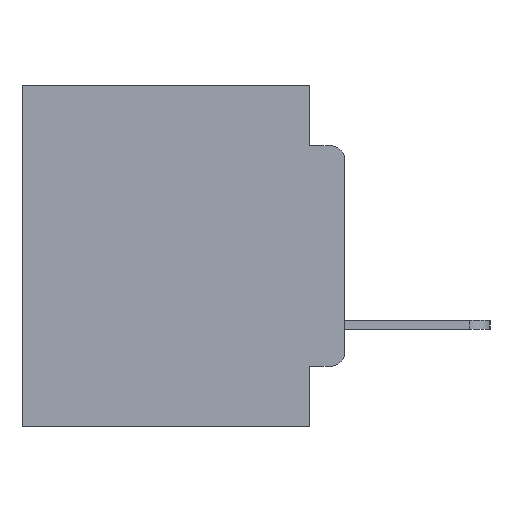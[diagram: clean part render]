
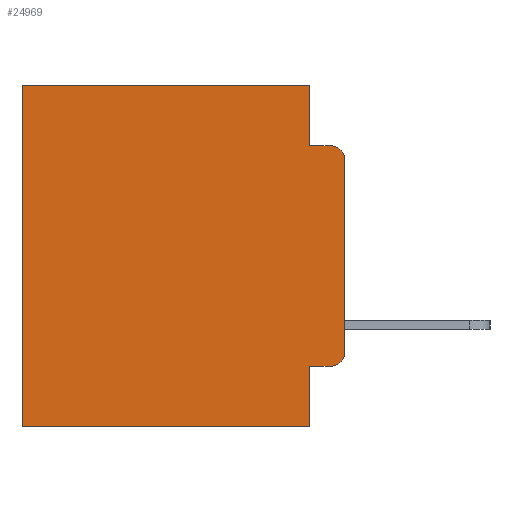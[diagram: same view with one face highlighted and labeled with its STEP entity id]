
A CAD part, left-side view. The second image highlights one B-rep face of the part: STEP entity #24969.
In plain terms, the highlighted planar face has unit normal (-1, 0, 0).
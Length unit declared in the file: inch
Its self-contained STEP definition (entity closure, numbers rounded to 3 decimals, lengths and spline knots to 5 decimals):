
#484 = CARTESIAN_POINT ( 'NONE',  ( 0.298, 0., -0.3915 ) ) ;
#609 = LINE ( 'NONE', #15113, #22962 ) ;
#954 = ORIENTED_EDGE ( 'NONE', *, *, #9728, .F. ) ;
#973 = CARTESIAN_POINT ( 'NONE',  ( 0.298, 0., 0. ) ) ;
#975 = EDGE_CURVE ( 'NONE', #1327, #17367, #3357, .T. ) ;
#1094 = LINE ( 'NONE', #25729, #12851 ) ;
#1327 = VERTEX_POINT ( 'NONE', #2108 ) ;
#1546 = CARTESIAN_POINT ( 'NONE',  ( 0.298, 0.051, -0.0885 ) ) ;
#2009 = EDGE_CURVE ( 'NONE', #8742, #11650, #5872, .T. ) ;
#2108 = CARTESIAN_POINT ( 'NONE',  ( 0.298, 0.473, 0. ) ) ;
#2180 = DIRECTION ( 'NONE',  ( -1., 0., 0. ) ) ;
#2583 = EDGE_CURVE ( 'NONE', #17834, #11650, #7219, .T. ) ;
#2671 = VECTOR ( 'NONE', #15167, 39.37008 ) ;
#2729 = VECTOR ( 'NONE', #8973, 39.37008 ) ;
#2906 = EDGE_CURVE ( 'NONE', #24728, #1327, #5493, .T. ) ;
#3357 = LINE ( 'NONE', #18942, #2729 ) ;
#3561 = ORIENTED_EDGE ( 'NONE', *, *, #2906, .T. ) ;
#4038 = CARTESIAN_POINT ( 'NONE',  ( 0.298, 0.051, -0.4115 ) ) ;
#5493 = LINE ( 'NONE', #973, #15902 ) ;
#5729 = DIRECTION ( 'NONE',  ( 0., 0., -1. ) ) ;
#5872 = LINE ( 'NONE', #25750, #15627 ) ;
#6986 = EDGE_LOOP ( 'NONE', ( #23642, #17729, #954, #14649, #3561, #11754, #18339, #25602, #8555, #21594 ) ) ;
#7070 = DIRECTION ( 'NONE',  ( 1., 0., 0. ) ) ;
#7219 = CIRCLE ( 'NONE', #7314, 0.02 ) ;
#7314 = AXIS2_PLACEMENT_3D ( 'NONE', #21985, #21525, #8734 ) ;
#8555 = ORIENTED_EDGE ( 'NONE', *, *, #23397, .T. ) ;
#8585 = DIRECTION ( 'NONE',  ( 0., -1., 0. ) ) ;
#8734 = DIRECTION ( 'NONE',  ( 0., 0., -1. ) ) ;
#8742 = VERTEX_POINT ( 'NONE', #20055 ) ;
#8872 = CARTESIAN_POINT ( 'NONE',  ( 0.298, 0.051, 0. ) ) ;
#8973 = DIRECTION ( 'NONE',  ( 0., 0., -1. ) ) ;
#9070 = EDGE_CURVE ( 'NONE', #24728, #11691, #13868, .T. ) ;
#9728 = EDGE_CURVE ( 'NONE', #11691, #14777, #12380, .T. ) ;
#11650 = VERTEX_POINT ( 'NONE', #484 ) ;
#11691 = VERTEX_POINT ( 'NONE', #25929 ) ;
#11754 = ORIENTED_EDGE ( 'NONE', *, *, #975, .T. ) ;
#12145 = DIRECTION ( 'NONE',  ( 0., 0., -1. ) ) ;
#12380 = LINE ( 'NONE', #1546, #22960 ) ;
#12495 = CARTESIAN_POINT ( 'NONE',  ( 0.298, 0.02, -0.0885 ) ) ;
#12851 = VECTOR ( 'NONE', #21689, 39.37008 ) ;
#13144 = CARTESIAN_POINT ( 'NONE',  ( 0.298, 0.051, -0.4115 ) ) ;
#13265 = VERTEX_POINT ( 'NONE', #4038 ) ;
#13487 = EDGE_CURVE ( 'NONE', #20129, #17367, #1094, .T. ) ;
#13746 = LINE ( 'NONE', #13144, #2671 ) ;
#13868 = LINE ( 'NONE', #8872, #19118 ) ;
#14029 = AXIS2_PLACEMENT_3D ( 'NONE', #19245, #7070, #21231 ) ;
#14601 = CARTESIAN_POINT ( 'NONE',  ( 0.298, 0.02, -0.1085 ) ) ;
#14649 = ORIENTED_EDGE ( 'NONE', *, *, #9070, .F. ) ;
#14777 = VERTEX_POINT ( 'NONE', #12495 ) ;
#15113 = CARTESIAN_POINT ( 'NONE',  ( 0.298, 0.051, 0. ) ) ;
#15167 = DIRECTION ( 'NONE',  ( 0., -1., 0. ) ) ;
#15296 = PLANE ( 'NONE',  #14029 ) ;
#15627 = VECTOR ( 'NONE', #12145, 39.37008 ) ;
#15902 = VECTOR ( 'NONE', #20746, 39.37008 ) ;
#16587 = DIRECTION ( 'NONE',  ( 0., 0., -1. ) ) ;
#16602 = CARTESIAN_POINT ( 'NONE',  ( 0.298, 0.051, 0. ) ) ;
#16802 = CARTESIAN_POINT ( 'NONE',  ( 0.298, 0.051, -0.5 ) ) ;
#16977 = EDGE_CURVE ( 'NONE', #13265, #20129, #609, .T. ) ;
#17367 = VERTEX_POINT ( 'NONE', #23023 ) ;
#17729 = ORIENTED_EDGE ( 'NONE', *, *, #21370, .T. ) ;
#17834 = VERTEX_POINT ( 'NONE', #20975 ) ;
#18201 = CIRCLE ( 'NONE', #18801, 0.02 ) ;
#18339 = ORIENTED_EDGE ( 'NONE', *, *, #13487, .F. ) ;
#18801 = AXIS2_PLACEMENT_3D ( 'NONE', #14601, #2180, #16587 ) ;
#18942 = CARTESIAN_POINT ( 'NONE',  ( 0.298, 0.473, 0. ) ) ;
#19118 = VECTOR ( 'NONE', #21144, 39.37008 ) ;
#19245 = CARTESIAN_POINT ( 'NONE',  ( 0.298, 0., 0. ) ) ;
#20055 = CARTESIAN_POINT ( 'NONE',  ( 0.298, 0., -0.1085 ) ) ;
#20129 = VERTEX_POINT ( 'NONE', #16802 ) ;
#20499 = FACE_OUTER_BOUND ( 'NONE', #6986, .T. ) ;
#20746 = DIRECTION ( 'NONE',  ( 0., 1., 0. ) ) ;
#20975 = CARTESIAN_POINT ( 'NONE',  ( 0.298, 0.02, -0.4115 ) ) ;
#21144 = DIRECTION ( 'NONE',  ( 0., 0., -1. ) ) ;
#21231 = DIRECTION ( 'NONE',  ( 0., 0., -1. ) ) ;
#21370 = EDGE_CURVE ( 'NONE', #8742, #14777, #18201, .T. ) ;
#21525 = DIRECTION ( 'NONE',  ( -1., 0., 0. ) ) ;
#21594 = ORIENTED_EDGE ( 'NONE', *, *, #2583, .T. ) ;
#21689 = DIRECTION ( 'NONE',  ( 0., 1., 0. ) ) ;
#21985 = CARTESIAN_POINT ( 'NONE',  ( 0.298, 0.02, -0.3915 ) ) ;
#22960 = VECTOR ( 'NONE', #8585, 39.37008 ) ;
#22962 = VECTOR ( 'NONE', #5729, 39.37008 ) ;
#23023 = CARTESIAN_POINT ( 'NONE',  ( 0.298, 0.473, -0.5 ) ) ;
#23397 = EDGE_CURVE ( 'NONE', #13265, #17834, #13746, .T. ) ;
#23642 = ORIENTED_EDGE ( 'NONE', *, *, #2009, .F. ) ;
#24728 = VERTEX_POINT ( 'NONE', #16602 ) ;
#24969 = ADVANCED_FACE ( 'NONE', ( #20499 ), #15296, .F. ) ;
#25602 = ORIENTED_EDGE ( 'NONE', *, *, #16977, .F. ) ;
#25729 = CARTESIAN_POINT ( 'NONE',  ( 0.298, 0., -0.5 ) ) ;
#25750 = CARTESIAN_POINT ( 'NONE',  ( 0.298, 0., 0. ) ) ;
#25929 = CARTESIAN_POINT ( 'NONE',  ( 0.298, 0.051, -0.0885 ) ) ;
